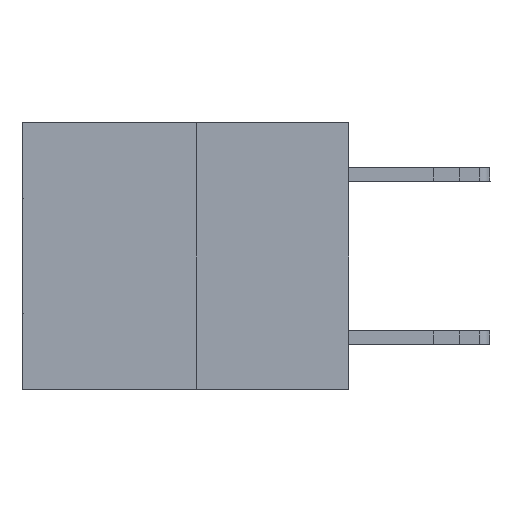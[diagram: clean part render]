
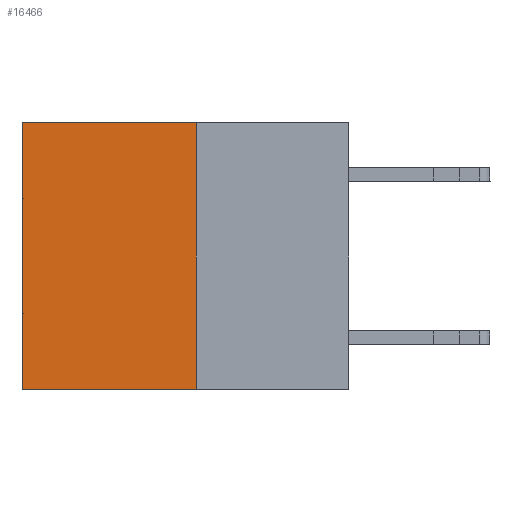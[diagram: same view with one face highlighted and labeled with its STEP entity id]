
A CAD part, left-side view. The second image highlights one B-rep face of the part: STEP entity #16466.
In plain terms, the highlighted planar face has unit normal (-1, 0, 0).
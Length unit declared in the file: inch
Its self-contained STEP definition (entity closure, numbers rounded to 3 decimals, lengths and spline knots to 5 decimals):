
#109 = FACE_OUTER_BOUND ( 'NONE', #11064, .T. ) ;
#795 = VECTOR ( 'NONE', #17248, 39.37008 ) ;
#6173 = LINE ( 'NONE', #7109, #28261 ) ;
#6499 = CARTESIAN_POINT ( 'NONE',  ( 0.3165, 0.6, -0.49 ) ) ;
#7036 = DIRECTION ( 'NONE',  ( 1., 0., 0. ) ) ;
#7109 = CARTESIAN_POINT ( 'NONE',  ( 0.3165, 0.6, -0.49 ) ) ;
#7771 = VERTEX_POINT ( 'NONE', #6499 ) ;
#8040 = VERTEX_POINT ( 'NONE', #30767 ) ;
#8847 = EDGE_CURVE ( 'NONE', #24418, #8040, #27452, .T. ) ;
#9868 = CARTESIAN_POINT ( 'NONE',  ( 0.3165, 0.28, -0.49 ) ) ;
#10844 = EDGE_CURVE ( 'NONE', #31471, #7771, #11793, .T. ) ;
#11064 = EDGE_LOOP ( 'NONE', ( #16605, #14685, #23338, #15058 ) ) ;
#11272 = CARTESIAN_POINT ( 'NONE',  ( 0.3165, 0.28, -0.49 ) ) ;
#11793 = LINE ( 'NONE', #9868, #19944 ) ;
#14217 = VECTOR ( 'NONE', #16990, 39.37008 ) ;
#14685 = ORIENTED_EDGE ( 'NONE', *, *, #10844, .F. ) ;
#15058 = ORIENTED_EDGE ( 'NONE', *, *, #8847, .T. ) ;
#16141 = PLANE ( 'NONE',  #25849 ) ;
#16466 = ADVANCED_FACE ( 'NONE', ( #109 ), #16141, .F. ) ;
#16605 = ORIENTED_EDGE ( 'NONE', *, *, #26577, .T. ) ;
#16990 = DIRECTION ( 'NONE',  ( 0., 1., 0. ) ) ;
#17248 = DIRECTION ( 'NONE',  ( 0., 0., -1. ) ) ;
#18989 = LINE ( 'NONE', #29736, #795 ) ;
#19149 = CARTESIAN_POINT ( 'NONE',  ( 0.3165, 0.28, 0. ) ) ;
#19944 = VECTOR ( 'NONE', #22420, 39.37008 ) ;
#22420 = DIRECTION ( 'NONE',  ( 0., 1., 0. ) ) ;
#23338 = ORIENTED_EDGE ( 'NONE', *, *, #26024, .F. ) ;
#24387 = DIRECTION ( 'NONE',  ( 0., 0., -1. ) ) ;
#24418 = VERTEX_POINT ( 'NONE', #19149 ) ;
#25849 = AXIS2_PLACEMENT_3D ( 'NONE', #11272, #7036, #24387 ) ;
#26024 = EDGE_CURVE ( 'NONE', #24418, #31471, #18989, .T. ) ;
#26577 = EDGE_CURVE ( 'NONE', #8040, #7771, #6173, .T. ) ;
#27452 = LINE ( 'NONE', #29395, #14217 ) ;
#28261 = VECTOR ( 'NONE', #29208, 39.37008 ) ;
#29208 = DIRECTION ( 'NONE',  ( 0., 0., -1. ) ) ;
#29395 = CARTESIAN_POINT ( 'NONE',  ( 0.3165, 0.28, 0. ) ) ;
#29736 = CARTESIAN_POINT ( 'NONE',  ( 0.3165, 0.28, -0.49 ) ) ;
#30589 = CARTESIAN_POINT ( 'NONE',  ( 0.3165, 0.28, -0.49 ) ) ;
#30767 = CARTESIAN_POINT ( 'NONE',  ( 0.3165, 0.6, 0. ) ) ;
#31471 = VERTEX_POINT ( 'NONE', #30589 ) ;
